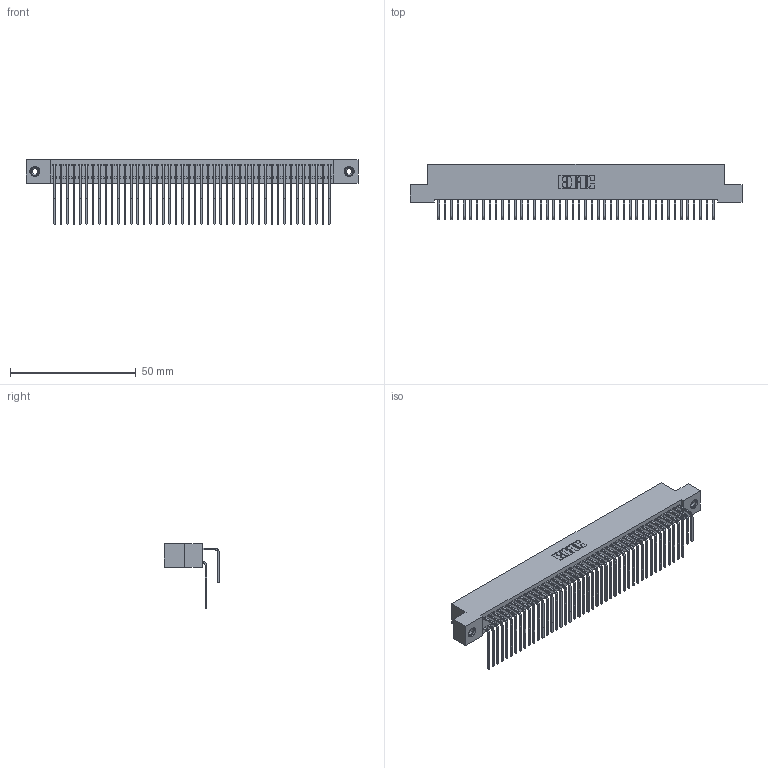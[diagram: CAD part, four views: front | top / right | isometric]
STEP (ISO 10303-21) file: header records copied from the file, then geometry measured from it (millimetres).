
FILE_DESCRIPTION (( 'STEP AP203' ), '1' );
FILE_NAME ('342-088-558-208.STEP', '2018-08-14T00:42:28', ( '' ), ( '' ), 'SwSTEP 2.0', 'SolidWorks 2016', '' );
FILE_SCHEMA (( 'CONFIG_CONTROL_DESIGN' ));
Length unit declared in the file: inch
Products named in the file (5): 342 Part_TI; 345-292-001_558 559 Tail - 1; 345-292-001_558 Tail - 2; 345-250-001_345-250-003-102; 342-088-558-208
Assembly tree (91 placements, depth 2):
  342-088-558-208
    342 Part_TI
    345-292-001_558 559 Tail - 1  x44
    345-292-001_558 Tail - 2  x44
    345-250-001_345-250-003-102  x2
Bounding box: 132.08 x 21.91 x 25.78 mm (x, y, z)
Volume: 12378.8 mm3; surface area: 22505.6 mm2
Topology: 91 solids, 91 shells, 4922 faces, 14603 edges, 9610 vertices
Faces by surface type: plane 3442, cylinder 1464, cone 12, torus 4
Entity records: 30886 total; most frequent: CARTESIAN_POINT 5148, ORIENTED_EDGE 5026, DIRECTION 4407, EDGE_CURVE 2513, LINE 2325, VECTOR 2325, VERTEX_POINT 1668, AXIS2_PLACEMENT_3D 1041
